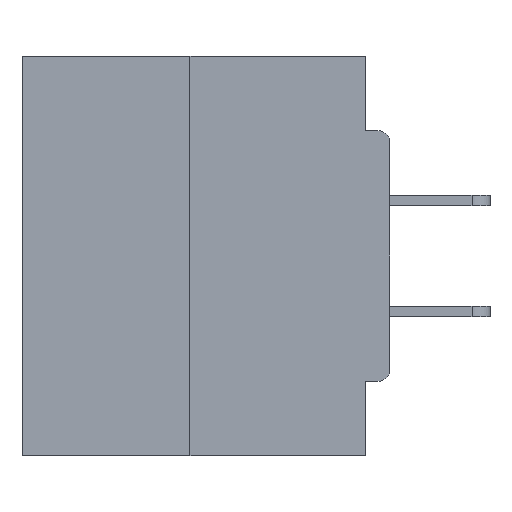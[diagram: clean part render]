
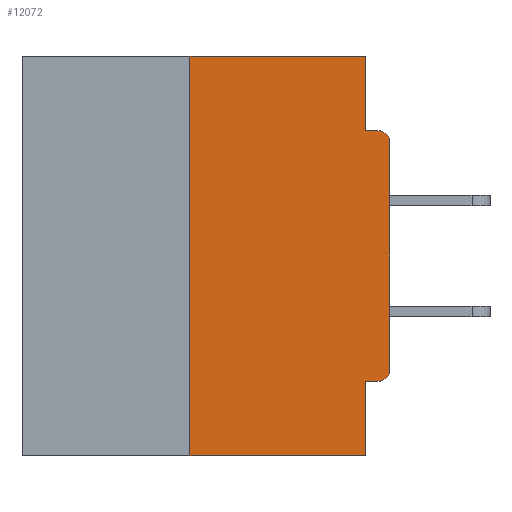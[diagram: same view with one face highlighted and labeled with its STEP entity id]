
A CAD part, left-side view. The second image highlights one B-rep face of the part: STEP entity #12072.
In plain terms, the highlighted planar face has unit normal (-1, 0, 0).
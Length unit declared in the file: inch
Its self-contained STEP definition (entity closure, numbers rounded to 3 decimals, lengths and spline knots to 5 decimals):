
#667 = VERTEX_POINT ( 'NONE', #17179 ) ;
#727 = CARTESIAN_POINT ( 'NONE',  ( 0., 0., -0.1085 ) ) ;
#1209 = DIRECTION ( 'NONE',  ( 0., 0., -1. ) ) ;
#2408 = CARTESIAN_POINT ( 'NONE',  ( 0., 0.46, 0. ) ) ;
#2417 = ORIENTED_EDGE ( 'NONE', *, *, #27097, .F. ) ;
#3129 = ORIENTED_EDGE ( 'NONE', *, *, #9165, .T. ) ;
#3233 = CARTESIAN_POINT ( 'NONE',  ( 0., 0., -0.0935 ) ) ;
#3305 = ORIENTED_EDGE ( 'NONE', *, *, #21865, .F. ) ;
#3321 = LINE ( 'NONE', #8190, #7560 ) ;
#3874 = VECTOR ( 'NONE', #31899, 39.37008 ) ;
#4136 = CARTESIAN_POINT ( 'NONE',  ( 0., 0.015, -0.1085 ) ) ;
#4333 = ORIENTED_EDGE ( 'NONE', *, *, #18810, .F. ) ;
#4388 = VERTEX_POINT ( 'NONE', #22385 ) ;
#4410 = DIRECTION ( 'NONE',  ( 0., 0., -1. ) ) ;
#4734 = EDGE_CURVE ( 'NONE', #12990, #4388, #12699, .T. ) ;
#4762 = VECTOR ( 'NONE', #23592, 39.37008 ) ;
#5619 = DIRECTION ( 'NONE',  ( 0., 0., -1. ) ) ;
#5803 = LINE ( 'NONE', #27716, #23931 ) ;
#6771 = VECTOR ( 'NONE', #11886, 39.37008 ) ;
#6829 = CARTESIAN_POINT ( 'NONE',  ( 0., 0.015, -0.4065 ) ) ;
#7528 = CARTESIAN_POINT ( 'NONE',  ( 0., 0.031, -0.4065 ) ) ;
#7560 = VECTOR ( 'NONE', #18217, 39.37008 ) ;
#8190 = CARTESIAN_POINT ( 'NONE',  ( 0., 0.25, 0. ) ) ;
#8980 = DIRECTION ( 'NONE',  ( -1., 0., 0. ) ) ;
#9165 = EDGE_CURVE ( 'NONE', #26027, #15308, #14799, .T. ) ;
#9234 = EDGE_CURVE ( 'NONE', #18437, #667, #9792, .T. ) ;
#9792 = CIRCLE ( 'NONE', #24228, 0.015 ) ;
#9878 = VERTEX_POINT ( 'NONE', #7528 ) ;
#10104 = ORIENTED_EDGE ( 'NONE', *, *, #15544, .F. ) ;
#10561 = DIRECTION ( 'NONE',  ( 0., -1., 0. ) ) ;
#10611 = EDGE_CURVE ( 'NONE', #667, #12990, #5803, .T. ) ;
#10892 = VERTEX_POINT ( 'NONE', #23938 ) ;
#11309 = CARTESIAN_POINT ( 'NONE',  ( 0., 0.031, -0.0935 ) ) ;
#11886 = DIRECTION ( 'NONE',  ( 0., 0., -1. ) ) ;
#12072 = ADVANCED_FACE ( 'NONE', ( #18506 ), #22331, .F. ) ;
#12078 = CARTESIAN_POINT ( 'NONE',  ( 0., 0.031, -0.5 ) ) ;
#12699 = CIRCLE ( 'NONE', #27594, 0.015 ) ;
#12701 = CARTESIAN_POINT ( 'NONE',  ( 0., 0., -0.4065 ) ) ;
#12990 = VERTEX_POINT ( 'NONE', #727 ) ;
#13286 = ORIENTED_EDGE ( 'NONE', *, *, #4734, .T. ) ;
#14126 = CARTESIAN_POINT ( 'NONE',  ( 0., 0.46, -0.5 ) ) ;
#14209 = ORIENTED_EDGE ( 'NONE', *, *, #23356, .F. ) ;
#14324 = CARTESIAN_POINT ( 'NONE',  ( 0., 0.46, 0. ) ) ;
#14449 = CARTESIAN_POINT ( 'NONE',  ( 0., 0.031, -0.5 ) ) ;
#14799 = LINE ( 'NONE', #14126, #4762 ) ;
#14894 = DIRECTION ( 'NONE',  ( 1., 0., 0. ) ) ;
#15308 = VERTEX_POINT ( 'NONE', #12078 ) ;
#15544 = EDGE_CURVE ( 'NONE', #18437, #9878, #25156, .T. ) ;
#16893 = CARTESIAN_POINT ( 'NONE',  ( 0., 0.031, 0. ) ) ;
#16921 = VECTOR ( 'NONE', #10561, 39.37008 ) ;
#17179 = CARTESIAN_POINT ( 'NONE',  ( 0., 0., -0.3915 ) ) ;
#17441 = VERTEX_POINT ( 'NONE', #11309 ) ;
#17631 = VERTEX_POINT ( 'NONE', #16893 ) ;
#18048 = DIRECTION ( 'NONE',  ( 0., 0., 1. ) ) ;
#18183 = CARTESIAN_POINT ( 'NONE',  ( 0., 0.25, -0.5 ) ) ;
#18217 = DIRECTION ( 'NONE',  ( 0., 0., 1. ) ) ;
#18437 = VERTEX_POINT ( 'NONE', #6829 ) ;
#18506 = FACE_OUTER_BOUND ( 'NONE', #23360, .T. ) ;
#18593 = VECTOR ( 'NONE', #5619, 39.37008 ) ;
#18744 = LINE ( 'NONE', #14449, #6771 ) ;
#18810 = EDGE_CURVE ( 'NONE', #26027, #10892, #3321, .T. ) ;
#20233 = DIRECTION ( 'NONE',  ( 0., 1., 0. ) ) ;
#21865 = EDGE_CURVE ( 'NONE', #10892, #17631, #26230, .T. ) ;
#22331 = PLANE ( 'NONE',  #30276 ) ;
#22385 = CARTESIAN_POINT ( 'NONE',  ( 0., 0.015, -0.0935 ) ) ;
#23063 = ORIENTED_EDGE ( 'NONE', *, *, #9234, .T. ) ;
#23077 = CARTESIAN_POINT ( 'NONE',  ( 0., 0.031, 0. ) ) ;
#23356 = EDGE_CURVE ( 'NONE', #17441, #4388, #24976, .T. ) ;
#23360 = EDGE_LOOP ( 'NONE', ( #3305, #4333, #3129, #2417, #10104, #23063, #31490, #13286, #14209, #23629 ) ) ;
#23574 = LINE ( 'NONE', #23077, #18593 ) ;
#23592 = DIRECTION ( 'NONE',  ( 0., -1., 0. ) ) ;
#23629 = ORIENTED_EDGE ( 'NONE', *, *, #30282, .F. ) ;
#23633 = DIRECTION ( 'NONE',  ( 0., 0., -1. ) ) ;
#23931 = VECTOR ( 'NONE', #18048, 39.37008 ) ;
#23938 = CARTESIAN_POINT ( 'NONE',  ( 0., 0.25, 0. ) ) ;
#24228 = AXIS2_PLACEMENT_3D ( 'NONE', #24343, #29093, #4410 ) ;
#24343 = CARTESIAN_POINT ( 'NONE',  ( 0., 0.015, -0.3915 ) ) ;
#24976 = LINE ( 'NONE', #3233, #16921 ) ;
#25156 = LINE ( 'NONE', #12701, #30961 ) ;
#26027 = VERTEX_POINT ( 'NONE', #18183 ) ;
#26230 = LINE ( 'NONE', #14324, #3874 ) ;
#27097 = EDGE_CURVE ( 'NONE', #9878, #15308, #18744, .T. ) ;
#27594 = AXIS2_PLACEMENT_3D ( 'NONE', #4136, #8980, #23633 ) ;
#27716 = CARTESIAN_POINT ( 'NONE',  ( 0., 0., 0. ) ) ;
#29093 = DIRECTION ( 'NONE',  ( -1., 0., 0. ) ) ;
#30276 = AXIS2_PLACEMENT_3D ( 'NONE', #2408, #14894, #1209 ) ;
#30282 = EDGE_CURVE ( 'NONE', #17631, #17441, #23574, .T. ) ;
#30961 = VECTOR ( 'NONE', #20233, 39.37008 ) ;
#31490 = ORIENTED_EDGE ( 'NONE', *, *, #10611, .T. ) ;
#31899 = DIRECTION ( 'NONE',  ( 0., -1., 0. ) ) ;
